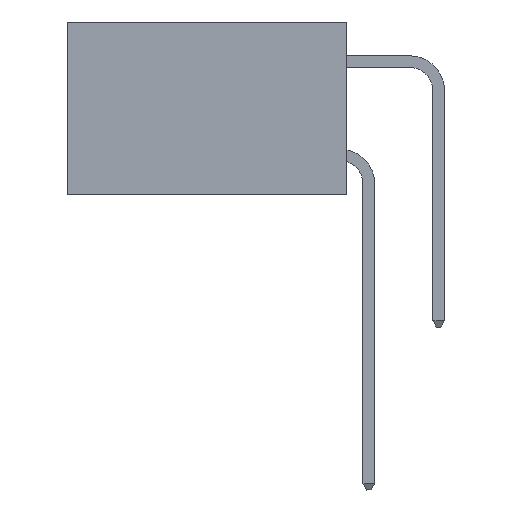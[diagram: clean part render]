
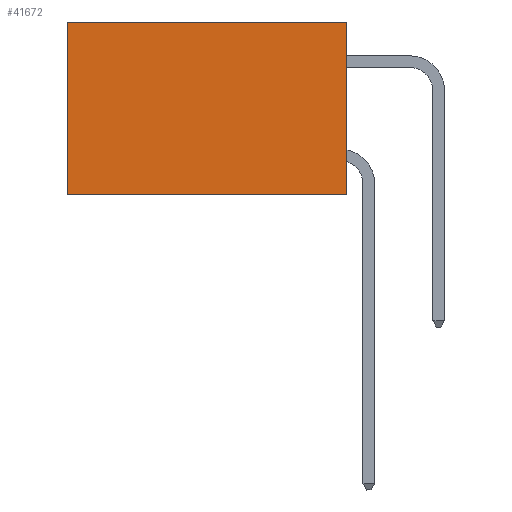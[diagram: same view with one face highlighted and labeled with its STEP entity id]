
A CAD part, left-side view. The second image highlights one B-rep face of the part: STEP entity #41672.
In plain terms, the highlighted planar face has unit normal (-1, 0, 0).
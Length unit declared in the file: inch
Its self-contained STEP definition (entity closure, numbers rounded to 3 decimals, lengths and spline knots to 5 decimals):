
#174 = DIRECTION ( 'NONE',  ( 1., 0., 0. ) ) ;
#181 = EDGE_CURVE ( 'NONE', #32752, #8618, #37521, .T. ) ;
#423 = VERTEX_POINT ( 'NONE', #19750 ) ;
#727 = LINE ( 'NONE', #13438, #42861 ) ;
#1182 = EDGE_CURVE ( 'NONE', #7491, #32752, #35868, .T. ) ;
#2565 = CARTESIAN_POINT ( 'NONE',  ( 0.2875, 0.6, -0.37 ) ) ;
#3786 = DIRECTION ( 'NONE',  ( 0., 1., 0. ) ) ;
#7053 = VECTOR ( 'NONE', #11432, 39.37008 ) ;
#7491 = VERTEX_POINT ( 'NONE', #41639 ) ;
#8618 = VERTEX_POINT ( 'NONE', #2565 ) ;
#10567 = ORIENTED_EDGE ( 'NONE', *, *, #181, .F. ) ;
#10651 = EDGE_CURVE ( 'NONE', #7491, #423, #727, .T. ) ;
#11432 = DIRECTION ( 'NONE',  ( 0., 1., 0. ) ) ;
#13438 = CARTESIAN_POINT ( 'NONE',  ( 0.2875, 0., 0. ) ) ;
#15340 = DIRECTION ( 'NONE',  ( 0., 0., -1. ) ) ;
#17022 = LINE ( 'NONE', #19306, #40690 ) ;
#18950 = DIRECTION ( 'NONE',  ( 0., 0., -1. ) ) ;
#19306 = CARTESIAN_POINT ( 'NONE',  ( 0.2875, 0.6, 0. ) ) ;
#19750 = CARTESIAN_POINT ( 'NONE',  ( 0.2875, 0.6, 0. ) ) ;
#22743 = CARTESIAN_POINT ( 'NONE',  ( 0.2875, 0., -0.37 ) ) ;
#23631 = DIRECTION ( 'NONE',  ( 0., 0., -1. ) ) ;
#27372 = ORIENTED_EDGE ( 'NONE', *, *, #1182, .F. ) ;
#27425 = EDGE_CURVE ( 'NONE', #423, #8618, #17022, .T. ) ;
#32752 = VERTEX_POINT ( 'NONE', #22743 ) ;
#32954 = ORIENTED_EDGE ( 'NONE', *, *, #27425, .T. ) ;
#33734 = VECTOR ( 'NONE', #18950, 39.37008 ) ;
#35868 = LINE ( 'NONE', #40691, #33734 ) ;
#36199 = CARTESIAN_POINT ( 'NONE',  ( 0.2875, 0., 0. ) ) ;
#37521 = LINE ( 'NONE', #38060, #7053 ) ;
#37960 = ORIENTED_EDGE ( 'NONE', *, *, #10651, .T. ) ;
#38060 = CARTESIAN_POINT ( 'NONE',  ( 0.2875, 0., -0.37 ) ) ;
#38775 = AXIS2_PLACEMENT_3D ( 'NONE', #36199, #174, #23631 ) ;
#39950 = PLANE ( 'NONE',  #38775 ) ;
#40690 = VECTOR ( 'NONE', #15340, 39.37008 ) ;
#40691 = CARTESIAN_POINT ( 'NONE',  ( 0.2875, 0., 0. ) ) ;
#41639 = CARTESIAN_POINT ( 'NONE',  ( 0.2875, 0., 0. ) ) ;
#41672 = ADVANCED_FACE ( 'NONE', ( #42774 ), #39950, .F. ) ;
#42774 = FACE_OUTER_BOUND ( 'NONE', #42952, .T. ) ;
#42861 = VECTOR ( 'NONE', #3786, 39.37008 ) ;
#42952 = EDGE_LOOP ( 'NONE', ( #32954, #10567, #27372, #37960 ) ) ;
